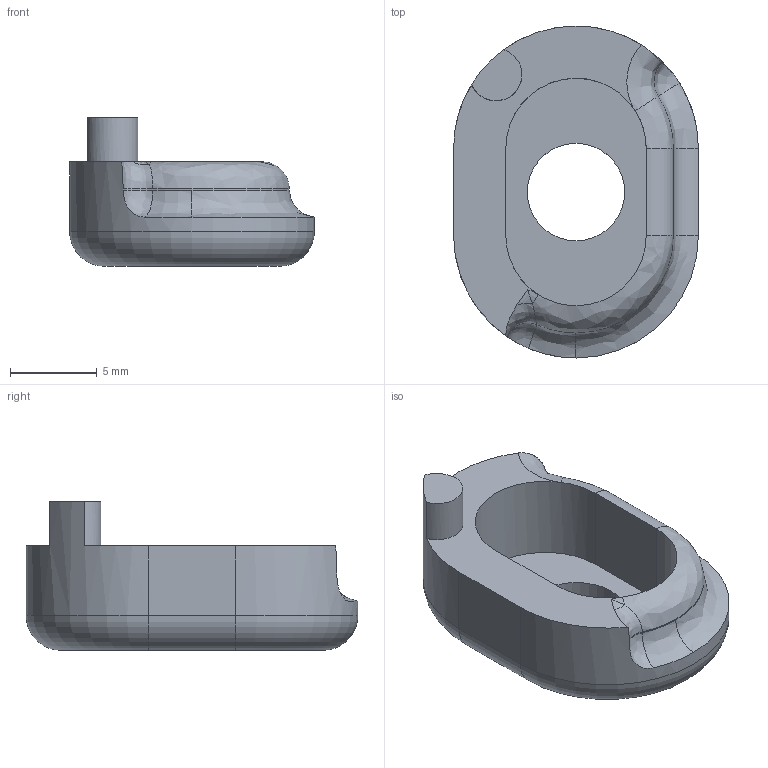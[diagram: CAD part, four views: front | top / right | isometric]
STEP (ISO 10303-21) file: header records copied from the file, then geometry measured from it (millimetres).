
FILE_DESCRIPTION (( 'STEP AP214' ), '1' );
FILE_NAME ('Easy_Mode_Release_Cover.STEP', '2013-12-17T09:03:46', ( 'elpi' ), ( '' ), 'SwSTEP 2.0', 'SolidWorks 2013', '' );
FILE_SCHEMA (( 'AUTOMOTIVE_DESIGN' ));
Length unit declared in the file: millimetre
Products named in the file (1): Easy_Mode_Release_Cover
Bounding box: 14.08 x 19.08 x 8.54 mm (x, y, z)
Volume: 737.3 mm3; surface area: 859 mm2
Topology: 1 solids, 1 shells, 47 faces, 114 edges, 69 vertices
Faces by surface type: cylinder 23, bspline 11, plane 10, torus 3
Entity records: 1703 total; most frequent: CARTESIAN_POINT 613, ORIENTED_EDGE 228, DIRECTION 219, EDGE_CURVE 114, AXIS2_PLACEMENT_3D 91, VERTEX_POINT 69, CIRCLE 54, EDGE_LOOP 49
